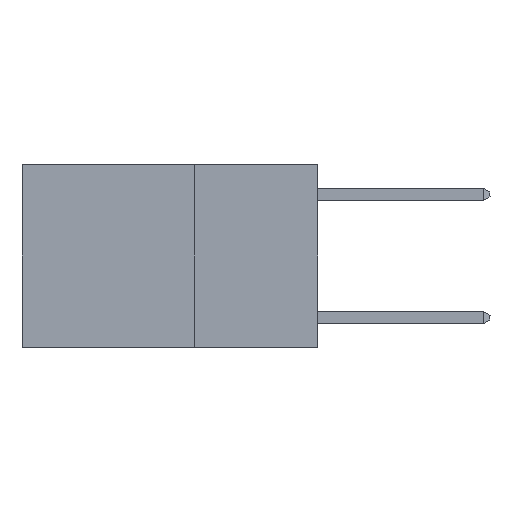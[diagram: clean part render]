
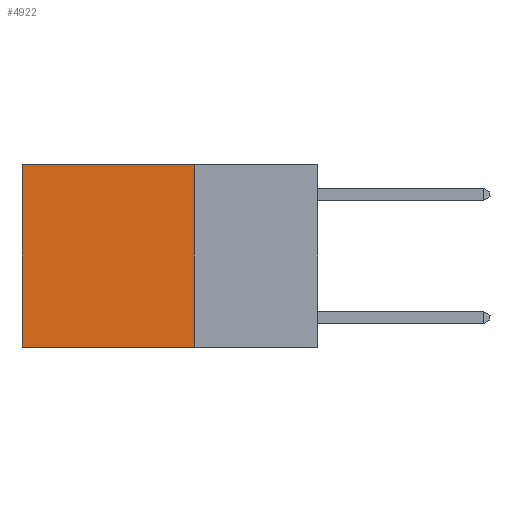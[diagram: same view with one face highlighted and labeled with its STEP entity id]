
A CAD part, left-side view. The second image highlights one B-rep face of the part: STEP entity #4922.
In plain terms, the highlighted planar face has unit normal (-1, 0, 0).
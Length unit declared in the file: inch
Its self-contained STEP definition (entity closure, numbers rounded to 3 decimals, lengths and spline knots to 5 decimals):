
#357 = DIRECTION ( 'NONE',  ( 0., 0., -1. ) ) ;
#957 = ORIENTED_EDGE ( 'NONE', *, *, #1953, .T. ) ;
#1331 = CARTESIAN_POINT ( 'NONE',  ( 0.2625, 0.25, -0.37 ) ) ;
#1641 = AXIS2_PLACEMENT_3D ( 'NONE', #6966, #1748, #3285 ) ;
#1748 = DIRECTION ( 'NONE',  ( 1., 0., 0. ) ) ;
#1898 = LINE ( 'NONE', #4820, #1938 ) ;
#1938 = VECTOR ( 'NONE', #357, 39.37008 ) ;
#1953 = EDGE_CURVE ( 'NONE', #5749, #3031, #4164, .T. ) ;
#2487 = EDGE_CURVE ( 'NONE', #2714, #5749, #6433, .T. ) ;
#2714 = VERTEX_POINT ( 'NONE', #5420 ) ;
#3031 = VERTEX_POINT ( 'NONE', #4570 ) ;
#3285 = DIRECTION ( 'NONE',  ( 0., 0., -1. ) ) ;
#3453 = DIRECTION ( 'NONE',  ( 0., 1., 0. ) ) ;
#3462 = DIRECTION ( 'NONE',  ( 0., 0., -1. ) ) ;
#3499 = LINE ( 'NONE', #1331, #9188 ) ;
#3756 = CARTESIAN_POINT ( 'NONE',  ( 0.2625, 0.6, 0. ) ) ;
#3996 = ORIENTED_EDGE ( 'NONE', *, *, #4624, .F. ) ;
#4164 = LINE ( 'NONE', #4852, #5182 ) ;
#4570 = CARTESIAN_POINT ( 'NONE',  ( 0.2625, 0.6, -0.37 ) ) ;
#4624 = EDGE_CURVE ( 'NONE', #2714, #6583, #1898, .T. ) ;
#4820 = CARTESIAN_POINT ( 'NONE',  ( 0.2625, 0.25, 0. ) ) ;
#4852 = CARTESIAN_POINT ( 'NONE',  ( 0.2625, 0.6, 0. ) ) ;
#4922 = ADVANCED_FACE ( 'NONE', ( #8963 ), #8395, .F. ) ;
#5182 = VECTOR ( 'NONE', #3462, 39.37008 ) ;
#5208 = ORIENTED_EDGE ( 'NONE', *, *, #2487, .T. ) ;
#5420 = CARTESIAN_POINT ( 'NONE',  ( 0.2625, 0.25, 0. ) ) ;
#5529 = EDGE_CURVE ( 'NONE', #6583, #3031, #3499, .T. ) ;
#5749 = VERTEX_POINT ( 'NONE', #3756 ) ;
#6433 = LINE ( 'NONE', #8666, #8783 ) ;
#6554 = DIRECTION ( 'NONE',  ( 0., 1., 0. ) ) ;
#6583 = VERTEX_POINT ( 'NONE', #6967 ) ;
#6966 = CARTESIAN_POINT ( 'NONE',  ( 0.2625, 0.25, 0. ) ) ;
#6967 = CARTESIAN_POINT ( 'NONE',  ( 0.2625, 0.25, -0.37 ) ) ;
#7733 = ORIENTED_EDGE ( 'NONE', *, *, #5529, .F. ) ;
#8395 = PLANE ( 'NONE',  #1641 ) ;
#8666 = CARTESIAN_POINT ( 'NONE',  ( 0.2625, 0.25, 0. ) ) ;
#8783 = VECTOR ( 'NONE', #3453, 39.37008 ) ;
#8963 = FACE_OUTER_BOUND ( 'NONE', #8984, .T. ) ;
#8984 = EDGE_LOOP ( 'NONE', ( #957, #7733, #3996, #5208 ) ) ;
#9188 = VECTOR ( 'NONE', #6554, 39.37008 ) ;
